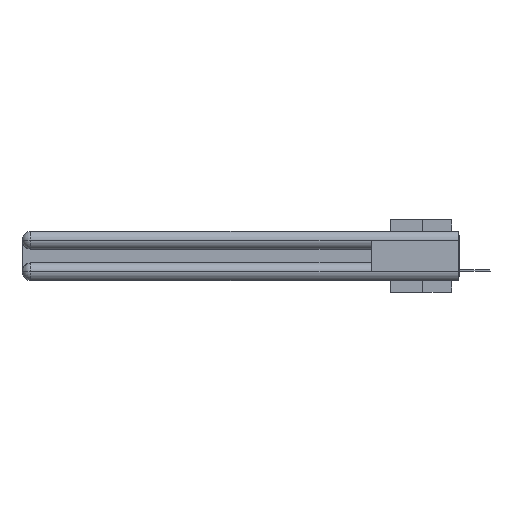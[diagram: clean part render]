
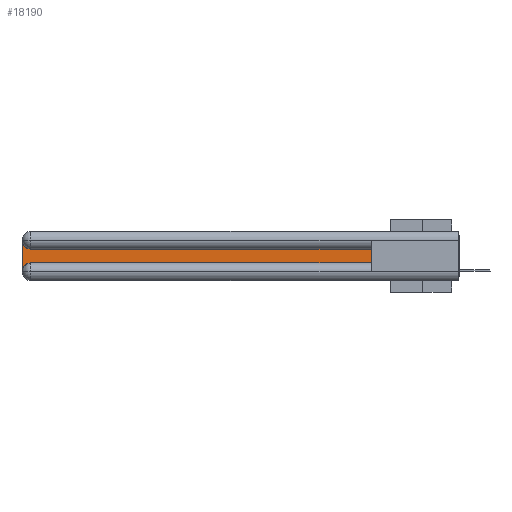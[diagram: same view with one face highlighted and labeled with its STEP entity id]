
A CAD part, left-side view. The second image highlights one B-rep face of the part: STEP entity #18190.
In plain terms, the highlighted planar face has unit normal (-1, 0, 0).
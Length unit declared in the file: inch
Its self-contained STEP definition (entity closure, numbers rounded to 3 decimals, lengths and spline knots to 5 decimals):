
#3362 = AXIS2_PLACEMENT_3D ( 'NONE', #36458, #24800, #24415 ) ;
#3448 = VERTEX_POINT ( 'NONE', #10163 ) ;
#4048 = ORIENTED_EDGE ( 'NONE', *, *, #19943, .T. ) ;
#4584 = CARTESIAN_POINT ( 'NONE',  ( 0.075, 0.6, -0.1225 ) ) ;
#5182 = DIRECTION ( 'NONE',  ( 1., 0., 0. ) ) ;
#5550 = DIRECTION ( 'NONE',  ( 0., 0., -1. ) ) ;
#5981 = EDGE_CURVE ( 'NONE', #29375, #3448, #9511, .T. ) ;
#6601 = CARTESIAN_POINT ( 'NONE',  ( 0.075, 3., -0.1225 ) ) ;
#6879 = DIRECTION ( 'NONE',  ( 1., 0., 0. ) ) ;
#7593 = CARTESIAN_POINT ( 'NONE',  ( 0.075, 2.94, -0.2175 ) ) ;
#8581 = ORIENTED_EDGE ( 'NONE', *, *, #12500, .T. ) ;
#8675 = ORIENTED_EDGE ( 'NONE', *, *, #10813, .T. ) ;
#9511 = LINE ( 'NONE', #19750, #22120 ) ;
#10163 = CARTESIAN_POINT ( 'NONE',  ( 0.075, 0.6, -0.2175 ) ) ;
#10513 = DIRECTION ( 'NONE',  ( 0., 1., 0. ) ) ;
#10813 = EDGE_CURVE ( 'NONE', #23675, #12378, #23167, .T. ) ;
#12378 = VERTEX_POINT ( 'NONE', #28477 ) ;
#12500 = EDGE_CURVE ( 'NONE', #3448, #25625, #27883, .T. ) ;
#13873 = ORIENTED_EDGE ( 'NONE', *, *, #5981, .T. ) ;
#13984 = VERTEX_POINT ( 'NONE', #31543 ) ;
#15837 = DIRECTION ( 'NONE',  ( 0., 0., -1. ) ) ;
#18190 = ADVANCED_FACE ( 'NONE', ( #31039 ), #24546, .F. ) ;
#18485 = EDGE_CURVE ( 'NONE', #13984, #29375, #20848, .T. ) ;
#19750 = CARTESIAN_POINT ( 'NONE',  ( 0.075, 0.6, -0.2175 ) ) ;
#19943 = EDGE_CURVE ( 'NONE', #25625, #23675, #28582, .T. ) ;
#20674 = VECTOR ( 'NONE', #10513, 39.37008 ) ;
#20848 = CIRCLE ( 'NONE', #3362, 0.06 ) ;
#21314 = CARTESIAN_POINT ( 'NONE',  ( 0.075, 0.6, -0.2175 ) ) ;
#21573 = CARTESIAN_POINT ( 'NONE',  ( 0.075, 2.94, -0.0625 ) ) ;
#22120 = VECTOR ( 'NONE', #34403, 39.37008 ) ;
#22404 = ORIENTED_EDGE ( 'NONE', *, *, #18485, .T. ) ;
#22997 = DIRECTION ( 'NONE',  ( 0., 0., -1. ) ) ;
#23167 = CIRCLE ( 'NONE', #33141, 0.06 ) ;
#23316 = EDGE_LOOP ( 'NONE', ( #4048, #8675, #29708, #22404, #13873, #8581 ) ) ;
#23589 = VECTOR ( 'NONE', #22997, 39.37008 ) ;
#23675 = VERTEX_POINT ( 'NONE', #35585 ) ;
#24134 = AXIS2_PLACEMENT_3D ( 'NONE', #6601, #5182, #5550 ) ;
#24415 = DIRECTION ( 'NONE',  ( 0., 0., -1. ) ) ;
#24546 = PLANE ( 'NONE',  #24134 ) ;
#24800 = DIRECTION ( 'NONE',  ( 1., 0., 0. ) ) ;
#25625 = VERTEX_POINT ( 'NONE', #30444 ) ;
#27317 = DIRECTION ( 'NONE',  ( 0., 0., 1. ) ) ;
#27883 = LINE ( 'NONE', #21314, #32467 ) ;
#28477 = CARTESIAN_POINT ( 'NONE',  ( 0.075, 3., -0.0625 ) ) ;
#28582 = LINE ( 'NONE', #4584, #20674 ) ;
#29375 = VERTEX_POINT ( 'NONE', #7593 ) ;
#29708 = ORIENTED_EDGE ( 'NONE', *, *, #37907, .T. ) ;
#30444 = CARTESIAN_POINT ( 'NONE',  ( 0.075, 0.6, -0.1225 ) ) ;
#31039 = FACE_OUTER_BOUND ( 'NONE', #23316, .T. ) ;
#31543 = CARTESIAN_POINT ( 'NONE',  ( 0.075, 3., -0.2775 ) ) ;
#32467 = VECTOR ( 'NONE', #27317, 39.37008 ) ;
#33141 = AXIS2_PLACEMENT_3D ( 'NONE', #21573, #6879, #15837 ) ;
#34403 = DIRECTION ( 'NONE',  ( 0., -1., 0. ) ) ;
#35218 = LINE ( 'NONE', #38041, #23589 ) ;
#35585 = CARTESIAN_POINT ( 'NONE',  ( 0.075, 2.94, -0.1225 ) ) ;
#36458 = CARTESIAN_POINT ( 'NONE',  ( 0.075, 2.94, -0.2775 ) ) ;
#37907 = EDGE_CURVE ( 'NONE', #12378, #13984, #35218, .T. ) ;
#38041 = CARTESIAN_POINT ( 'NONE',  ( 0.075, 3., -0.2175 ) ) ;
